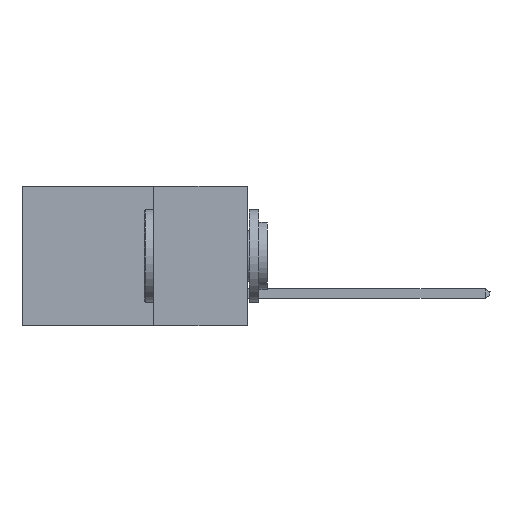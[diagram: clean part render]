
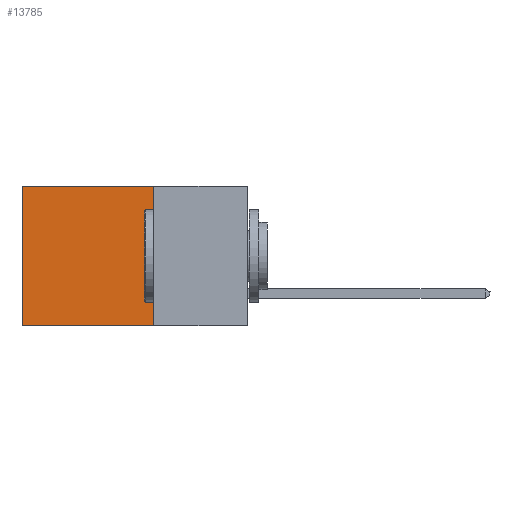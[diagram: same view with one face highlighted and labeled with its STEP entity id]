
A CAD part, left-side view. The second image highlights one B-rep face of the part: STEP entity #13785.
In plain terms, the highlighted planar face has unit normal (-1, 0, 0).
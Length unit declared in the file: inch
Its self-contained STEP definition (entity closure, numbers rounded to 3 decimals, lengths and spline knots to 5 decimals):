
#191 = DIRECTION ( 'NONE',  ( 0., 0., -1. ) ) ;
#624 = DIRECTION ( 'NONE',  ( 0., 1., 0. ) ) ;
#923 = CARTESIAN_POINT ( 'NONE',  ( 0.2615, 0.25, -0.37 ) ) ;
#1059 = EDGE_LOOP ( 'NONE', ( #1155, #1372, #14983, #8092 ) ) ;
#1117 = LINE ( 'NONE', #923, #6272 ) ;
#1155 = ORIENTED_EDGE ( 'NONE', *, *, #8983, .T. ) ;
#1372 = ORIENTED_EDGE ( 'NONE', *, *, #14306, .F. ) ;
#1778 = PLANE ( 'NONE',  #2057 ) ;
#2057 = AXIS2_PLACEMENT_3D ( 'NONE', #8056, #7865, #191 ) ;
#3259 = VERTEX_POINT ( 'NONE', #3567 ) ;
#3400 = VECTOR ( 'NONE', #9889, 39.37008 ) ;
#3567 = CARTESIAN_POINT ( 'NONE',  ( 0.2615, 0.6, -0.37 ) ) ;
#3741 = CARTESIAN_POINT ( 'NONE',  ( 0.2615, 0.6, 0. ) ) ;
#4411 = DIRECTION ( 'NONE',  ( 0., 0., -1. ) ) ;
#4557 = CARTESIAN_POINT ( 'NONE',  ( 0.2615, 0.25, -0.37 ) ) ;
#6196 = CARTESIAN_POINT ( 'NONE',  ( 0.2615, 0.25, 0. ) ) ;
#6272 = VECTOR ( 'NONE', #4411, 39.37008 ) ;
#6569 = FACE_OUTER_BOUND ( 'NONE', #1059, .T. ) ;
#7194 = DIRECTION ( 'NONE',  ( 0., 0., -1. ) ) ;
#7806 = CARTESIAN_POINT ( 'NONE',  ( 0.2615, 0.25, -0.37 ) ) ;
#7865 = DIRECTION ( 'NONE',  ( 1., 0., 0. ) ) ;
#8056 = CARTESIAN_POINT ( 'NONE',  ( 0.2615, 0.25, -0.37 ) ) ;
#8092 = ORIENTED_EDGE ( 'NONE', *, *, #8735, .T. ) ;
#8294 = CARTESIAN_POINT ( 'NONE',  ( 0.2615, 0.25, 0. ) ) ;
#8735 = EDGE_CURVE ( 'NONE', #18658, #16586, #17208, .T. ) ;
#8983 = EDGE_CURVE ( 'NONE', #16586, #3259, #16302, .T. ) ;
#9889 = DIRECTION ( 'NONE',  ( 0., 1., 0. ) ) ;
#10978 = LINE ( 'NONE', #7806, #15964 ) ;
#11086 = VERTEX_POINT ( 'NONE', #4557 ) ;
#13785 = ADVANCED_FACE ( 'NONE', ( #6569 ), #1778, .F. ) ;
#14306 = EDGE_CURVE ( 'NONE', #11086, #3259, #10978, .T. ) ;
#14721 = CARTESIAN_POINT ( 'NONE',  ( 0.2615, 0.6, -0.37 ) ) ;
#14983 = ORIENTED_EDGE ( 'NONE', *, *, #18463, .F. ) ;
#15964 = VECTOR ( 'NONE', #624, 39.37008 ) ;
#16302 = LINE ( 'NONE', #14721, #16713 ) ;
#16586 = VERTEX_POINT ( 'NONE', #3741 ) ;
#16713 = VECTOR ( 'NONE', #7194, 39.37008 ) ;
#17208 = LINE ( 'NONE', #8294, #3400 ) ;
#18463 = EDGE_CURVE ( 'NONE', #18658, #11086, #1117, .T. ) ;
#18658 = VERTEX_POINT ( 'NONE', #6196 ) ;
